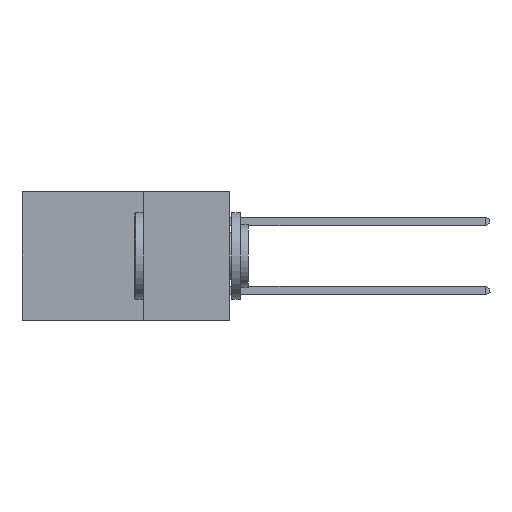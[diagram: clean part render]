
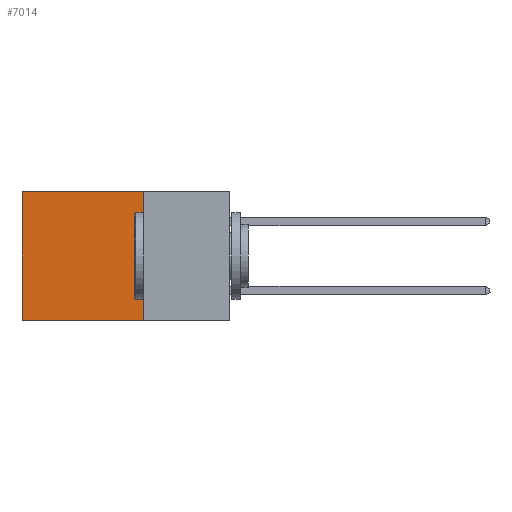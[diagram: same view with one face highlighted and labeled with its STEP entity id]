
A CAD part, left-side view. The second image highlights one B-rep face of the part: STEP entity #7014.
In plain terms, the highlighted planar face has unit normal (-1, 0, 0).
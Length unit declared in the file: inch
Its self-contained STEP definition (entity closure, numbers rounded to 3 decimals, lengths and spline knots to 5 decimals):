
#21 = DIRECTION ( 'NONE',  ( 0., 0., -1. ) ) ;
#83 = PLANE ( 'NONE',  #9432 ) ;
#147 = CARTESIAN_POINT ( 'NONE',  ( 0.298, 0.6, 0. ) ) ;
#557 = CARTESIAN_POINT ( 'NONE',  ( 0.298, 0.6, 0. ) ) ;
#709 = VERTEX_POINT ( 'NONE', #6131 ) ;
#851 = ORIENTED_EDGE ( 'NONE', *, *, #15596, .F. ) ;
#1351 = EDGE_CURVE ( 'NONE', #1656, #7027, #9657, .T. ) ;
#1656 = VERTEX_POINT ( 'NONE', #14439 ) ;
#3427 = LINE ( 'NONE', #9708, #13450 ) ;
#4132 = CARTESIAN_POINT ( 'NONE',  ( 0.298, 0.6, -0.37 ) ) ;
#5501 = DIRECTION ( 'NONE',  ( 0., 0., -1. ) ) ;
#5604 = ORIENTED_EDGE ( 'NONE', *, *, #11005, .T. ) ;
#5763 = CARTESIAN_POINT ( 'NONE',  ( 0.298, 0.25, 0. ) ) ;
#6131 = CARTESIAN_POINT ( 'NONE',  ( 0.298, 0.25, -0.37 ) ) ;
#6428 = VECTOR ( 'NONE', #21, 39.37008 ) ;
#7014 = ADVANCED_FACE ( 'NONE', ( #8746 ), #83, .F. ) ;
#7027 = VERTEX_POINT ( 'NONE', #147 ) ;
#7227 = DIRECTION ( 'NONE',  ( 1., 0., 0. ) ) ;
#7440 = VECTOR ( 'NONE', #5501, 39.37008 ) ;
#8161 = VECTOR ( 'NONE', #12615, 39.37008 ) ;
#8746 = FACE_OUTER_BOUND ( 'NONE', #11098, .T. ) ;
#9064 = CARTESIAN_POINT ( 'NONE',  ( 0.298, 0.25, 0. ) ) ;
#9432 = AXIS2_PLACEMENT_3D ( 'NONE', #13478, #7227, #12157 ) ;
#9657 = LINE ( 'NONE', #9064, #8161 ) ;
#9708 = CARTESIAN_POINT ( 'NONE',  ( 0.298, 0.25, -0.37 ) ) ;
#9870 = DIRECTION ( 'NONE',  ( 0., 1., 0. ) ) ;
#11005 = EDGE_CURVE ( 'NONE', #7027, #12536, #13893, .T. ) ;
#11098 = EDGE_LOOP ( 'NONE', ( #5604, #11673, #851, #15229 ) ) ;
#11673 = ORIENTED_EDGE ( 'NONE', *, *, #13034, .F. ) ;
#12157 = DIRECTION ( 'NONE',  ( 0., 0., -1. ) ) ;
#12536 = VERTEX_POINT ( 'NONE', #4132 ) ;
#12615 = DIRECTION ( 'NONE',  ( 0., 1., 0. ) ) ;
#12877 = LINE ( 'NONE', #5763, #6428 ) ;
#13034 = EDGE_CURVE ( 'NONE', #709, #12536, #3427, .T. ) ;
#13450 = VECTOR ( 'NONE', #9870, 39.37008 ) ;
#13478 = CARTESIAN_POINT ( 'NONE',  ( 0.298, 0.25, 0. ) ) ;
#13893 = LINE ( 'NONE', #557, #7440 ) ;
#14439 = CARTESIAN_POINT ( 'NONE',  ( 0.298, 0.25, 0. ) ) ;
#15229 = ORIENTED_EDGE ( 'NONE', *, *, #1351, .T. ) ;
#15596 = EDGE_CURVE ( 'NONE', #1656, #709, #12877, .T. ) ;
